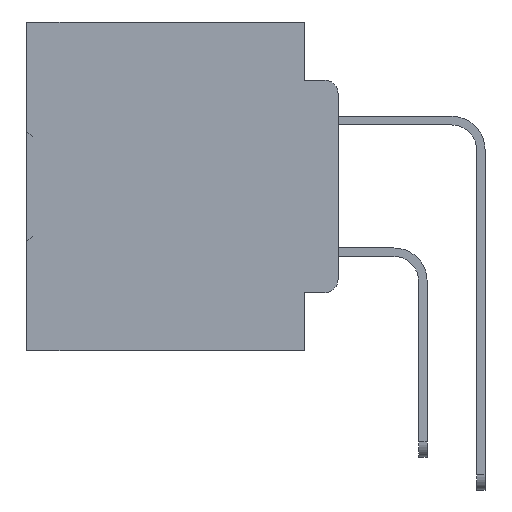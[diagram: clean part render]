
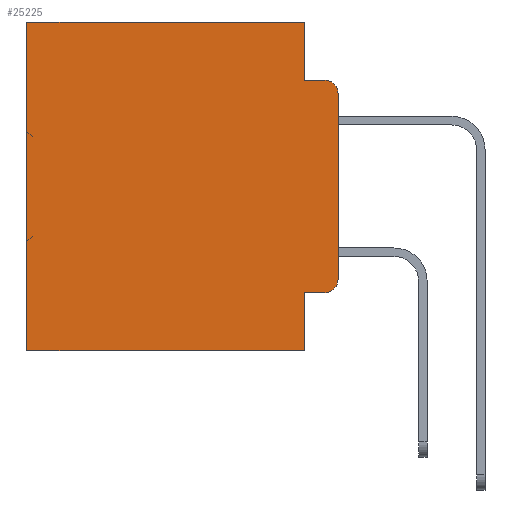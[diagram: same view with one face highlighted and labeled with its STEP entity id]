
A CAD part, left-side view. The second image highlights one B-rep face of the part: STEP entity #25225.
In plain terms, the highlighted planar face has unit normal (-1, 0, 0).
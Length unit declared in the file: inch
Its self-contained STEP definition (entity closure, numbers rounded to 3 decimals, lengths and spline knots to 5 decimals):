
#316 = LINE ( 'NONE', #7533, #22991 ) ;
#478 = AXIS2_PLACEMENT_3D ( 'NONE', #16745, #28972, #10674 ) ;
#740 = VERTEX_POINT ( 'NONE', #29088 ) ;
#965 = EDGE_CURVE ( 'NONE', #27410, #2641, #6176, .T. ) ;
#1054 = VERTEX_POINT ( 'NONE', #22056 ) ;
#2641 = VERTEX_POINT ( 'NONE', #3194 ) ;
#2824 = ORIENTED_EDGE ( 'NONE', *, *, #16369, .T. ) ;
#3194 = CARTESIAN_POINT ( 'NONE',  ( 0.298, 0.473, 0. ) ) ;
#3379 = DIRECTION ( 'NONE',  ( -1., 0., 0. ) ) ;
#3831 = CARTESIAN_POINT ( 'NONE',  ( 0.298, 0.473, 0. ) ) ;
#3960 = CARTESIAN_POINT ( 'NONE',  ( 0.298, 0.473, -0.5 ) ) ;
#4416 = VECTOR ( 'NONE', #33229, 39.37008 ) ;
#4952 = CARTESIAN_POINT ( 'NONE',  ( 0.298, 0.02, -0.3915 ) ) ;
#5517 = VERTEX_POINT ( 'NONE', #21760 ) ;
#6176 = LINE ( 'NONE', #28052, #14429 ) ;
#6429 = LINE ( 'NONE', #3831, #37900 ) ;
#7392 = CARTESIAN_POINT ( 'NONE',  ( 0.298, 0.051, 0. ) ) ;
#7533 = CARTESIAN_POINT ( 'NONE',  ( 0.298, 0.051, 0. ) ) ;
#7722 = ORIENTED_EDGE ( 'NONE', *, *, #11973, .F. ) ;
#8085 = DIRECTION ( 'NONE',  ( 0., 0., -1. ) ) ;
#9494 = CARTESIAN_POINT ( 'NONE',  ( 0.298, 0.02, -0.0885 ) ) ;
#10173 = ORIENTED_EDGE ( 'NONE', *, *, #10672, .F. ) ;
#10672 = EDGE_CURVE ( 'NONE', #25331, #32392, #12801, .T. ) ;
#10674 = DIRECTION ( 'NONE',  ( 0., 0., -1. ) ) ;
#11612 = ORIENTED_EDGE ( 'NONE', *, *, #35803, .T. ) ;
#11652 = ORIENTED_EDGE ( 'NONE', *, *, #15539, .F. ) ;
#11884 = CARTESIAN_POINT ( 'NONE',  ( 0.298, 0., 0. ) ) ;
#11973 = EDGE_CURVE ( 'NONE', #1054, #16800, #19870, .T. ) ;
#12801 = LINE ( 'NONE', #35766, #19983 ) ;
#13028 = ORIENTED_EDGE ( 'NONE', *, *, #39439, .F. ) ;
#13515 = ORIENTED_EDGE ( 'NONE', *, *, #25913, .F. ) ;
#14429 = VECTOR ( 'NONE', #28003, 39.37008 ) ;
#14544 = DIRECTION ( 'NONE',  ( 0., -1., 0. ) ) ;
#15539 = EDGE_CURVE ( 'NONE', #27410, #25331, #316, .T. ) ;
#16093 = VERTEX_POINT ( 'NONE', #22669 ) ;
#16344 = AXIS2_PLACEMENT_3D ( 'NONE', #21882, #3379, #24918 ) ;
#16369 = EDGE_CURVE ( 'NONE', #740, #16093, #18643, .T. ) ;
#16715 = VECTOR ( 'NONE', #26021, 39.37008 ) ;
#16745 = CARTESIAN_POINT ( 'NONE',  ( 0.298, 0., 0. ) ) ;
#16800 = VERTEX_POINT ( 'NONE', #26485 ) ;
#17102 = ORIENTED_EDGE ( 'NONE', *, *, #31371, .T. ) ;
#18304 = EDGE_CURVE ( 'NONE', #2641, #27906, #6429, .T. ) ;
#18643 = LINE ( 'NONE', #23967, #33877 ) ;
#19870 = LINE ( 'NONE', #11884, #4416 ) ;
#19983 = VECTOR ( 'NONE', #14544, 39.37008 ) ;
#20182 = EDGE_LOOP ( 'NONE', ( #7722, #11612, #10173, #11652, #30780, #36302, #13028, #13515, #2824, #17102 ) ) ;
#21760 = CARTESIAN_POINT ( 'NONE',  ( 0.298, 0.051, -0.5 ) ) ;
#21882 = CARTESIAN_POINT ( 'NONE',  ( 0.298, 0.02, -0.1085 ) ) ;
#22056 = CARTESIAN_POINT ( 'NONE',  ( 0.298, 0., -0.1085 ) ) ;
#22669 = CARTESIAN_POINT ( 'NONE',  ( 0.298, 0.02, -0.4115 ) ) ;
#22991 = VECTOR ( 'NONE', #38028, 39.37008 ) ;
#23967 = CARTESIAN_POINT ( 'NONE',  ( 0.298, 0.051, -0.4115 ) ) ;
#24918 = DIRECTION ( 'NONE',  ( 0., 0., -1. ) ) ;
#25225 = ADVANCED_FACE ( 'NONE', ( #38567 ), #25935, .F. ) ;
#25331 = VERTEX_POINT ( 'NONE', #35449 ) ;
#25751 = LINE ( 'NONE', #32013, #16715 ) ;
#25913 = EDGE_CURVE ( 'NONE', #740, #5517, #25751, .T. ) ;
#25935 = PLANE ( 'NONE',  #478 ) ;
#26021 = DIRECTION ( 'NONE',  ( 0., 0., -1. ) ) ;
#26443 = DIRECTION ( 'NONE',  ( -1., 0., 0. ) ) ;
#26485 = CARTESIAN_POINT ( 'NONE',  ( 0.298, 0., -0.3915 ) ) ;
#27044 = DIRECTION ( 'NONE',  ( 0., -1., 0. ) ) ;
#27410 = VERTEX_POINT ( 'NONE', #7392 ) ;
#27906 = VERTEX_POINT ( 'NONE', #3960 ) ;
#28003 = DIRECTION ( 'NONE',  ( 0., 1., 0. ) ) ;
#28052 = CARTESIAN_POINT ( 'NONE',  ( 0.298, 0., 0. ) ) ;
#28972 = DIRECTION ( 'NONE',  ( 1., 0., 0. ) ) ;
#29049 = CIRCLE ( 'NONE', #16344, 0.02 ) ;
#29088 = CARTESIAN_POINT ( 'NONE',  ( 0.298, 0.051, -0.4115 ) ) ;
#30780 = ORIENTED_EDGE ( 'NONE', *, *, #965, .T. ) ;
#30823 = CIRCLE ( 'NONE', #33312, 0.02 ) ;
#31371 = EDGE_CURVE ( 'NONE', #16093, #16800, #30823, .T. ) ;
#32013 = CARTESIAN_POINT ( 'NONE',  ( 0.298, 0.051, 0. ) ) ;
#32392 = VERTEX_POINT ( 'NONE', #9494 ) ;
#32746 = CARTESIAN_POINT ( 'NONE',  ( 0.298, 0., -0.5 ) ) ;
#33229 = DIRECTION ( 'NONE',  ( 0., 0., -1. ) ) ;
#33312 = AXIS2_PLACEMENT_3D ( 'NONE', #4952, #26443, #8085 ) ;
#33877 = VECTOR ( 'NONE', #27044, 39.37008 ) ;
#34504 = DIRECTION ( 'NONE',  ( 0., 0., -1. ) ) ;
#35449 = CARTESIAN_POINT ( 'NONE',  ( 0.298, 0.051, -0.0885 ) ) ;
#35551 = VECTOR ( 'NONE', #38750, 39.37008 ) ;
#35766 = CARTESIAN_POINT ( 'NONE',  ( 0.298, 0.051, -0.0885 ) ) ;
#35803 = EDGE_CURVE ( 'NONE', #1054, #32392, #29049, .T. ) ;
#36302 = ORIENTED_EDGE ( 'NONE', *, *, #18304, .T. ) ;
#36473 = LINE ( 'NONE', #32746, #35551 ) ;
#37900 = VECTOR ( 'NONE', #34504, 39.37008 ) ;
#38028 = DIRECTION ( 'NONE',  ( 0., 0., -1. ) ) ;
#38567 = FACE_OUTER_BOUND ( 'NONE', #20182, .T. ) ;
#38750 = DIRECTION ( 'NONE',  ( 0., 1., 0. ) ) ;
#39439 = EDGE_CURVE ( 'NONE', #5517, #27906, #36473, .T. ) ;
